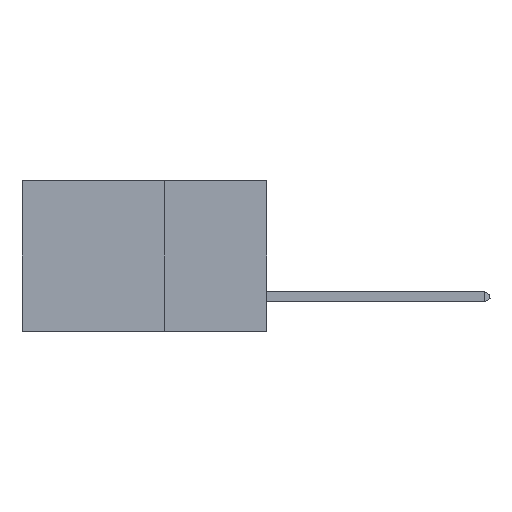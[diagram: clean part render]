
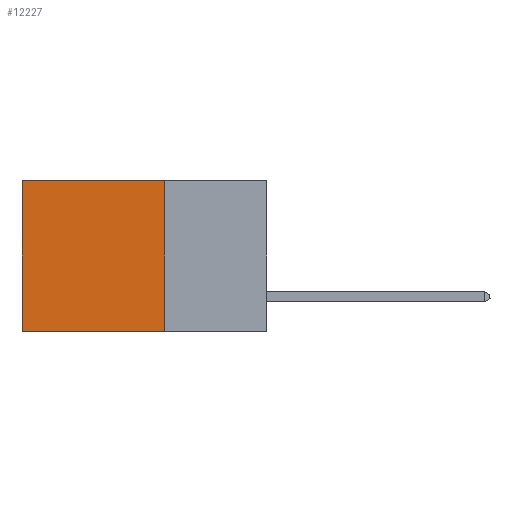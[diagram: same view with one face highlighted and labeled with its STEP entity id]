
A CAD part, left-side view. The second image highlights one B-rep face of the part: STEP entity #12227.
In plain terms, the highlighted planar face has unit normal (-1, 0, 0).
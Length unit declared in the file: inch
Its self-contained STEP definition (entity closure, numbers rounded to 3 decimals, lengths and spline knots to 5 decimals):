
#203 = ORIENTED_EDGE ( 'NONE', *, *, #2000, .F. ) ;
#1273 = ORIENTED_EDGE ( 'NONE', *, *, #4334, .T. ) ;
#1590 = VECTOR ( 'NONE', #4318, 39.37008 ) ;
#2000 = EDGE_CURVE ( 'NONE', #8468, #23145, #29877, .T. ) ;
#4318 = DIRECTION ( 'NONE',  ( 0., 1., 0. ) ) ;
#4334 = EDGE_CURVE ( 'NONE', #22499, #25801, #22245, .T. ) ;
#4381 = EDGE_LOOP ( 'NONE', ( #28928, #203, #22997, #1273 ) ) ;
#4832 = PLANE ( 'NONE',  #26429 ) ;
#5043 = VECTOR ( 'NONE', #27438, 39.37008 ) ;
#5474 = VECTOR ( 'NONE', #24535, 39.37008 ) ;
#6563 = CARTESIAN_POINT ( 'NONE',  ( 0.2875, 0.25, -0.37 ) ) ;
#7083 = DIRECTION ( 'NONE',  ( 0., 0., -1. ) ) ;
#8468 = VERTEX_POINT ( 'NONE', #30933 ) ;
#9014 = CARTESIAN_POINT ( 'NONE',  ( 0.2875, 0.6, -0.37 ) ) ;
#9348 = CARTESIAN_POINT ( 'NONE',  ( 0.2875, 0.25, 0. ) ) ;
#11976 = LINE ( 'NONE', #24220, #5474 ) ;
#12227 = ADVANCED_FACE ( 'NONE', ( #18623 ), #4832, .F. ) ;
#12377 = CARTESIAN_POINT ( 'NONE',  ( 0.2875, 0.25, 0. ) ) ;
#14038 = LINE ( 'NONE', #21580, #28235 ) ;
#14568 = EDGE_CURVE ( 'NONE', #22499, #8468, #11976, .T. ) ;
#15264 = CARTESIAN_POINT ( 'NONE',  ( 0.2875, 0.25, 0. ) ) ;
#16583 = EDGE_CURVE ( 'NONE', #25801, #23145, #14038, .T. ) ;
#18623 = FACE_OUTER_BOUND ( 'NONE', #4381, .T. ) ;
#21580 = CARTESIAN_POINT ( 'NONE',  ( 0.2875, 0.6, 0. ) ) ;
#22245 = LINE ( 'NONE', #12377, #5043 ) ;
#22499 = VERTEX_POINT ( 'NONE', #15264 ) ;
#22997 = ORIENTED_EDGE ( 'NONE', *, *, #14568, .F. ) ;
#23145 = VERTEX_POINT ( 'NONE', #9014 ) ;
#24220 = CARTESIAN_POINT ( 'NONE',  ( 0.2875, 0.25, 0. ) ) ;
#24535 = DIRECTION ( 'NONE',  ( 0., 0., -1. ) ) ;
#25192 = DIRECTION ( 'NONE',  ( 0., 0., -1. ) ) ;
#25801 = VERTEX_POINT ( 'NONE', #27856 ) ;
#26429 = AXIS2_PLACEMENT_3D ( 'NONE', #9348, #26432, #7083 ) ;
#26432 = DIRECTION ( 'NONE',  ( 1., 0., 0. ) ) ;
#27438 = DIRECTION ( 'NONE',  ( 0., 1., 0. ) ) ;
#27856 = CARTESIAN_POINT ( 'NONE',  ( 0.2875, 0.6, 0. ) ) ;
#28235 = VECTOR ( 'NONE', #25192, 39.37008 ) ;
#28928 = ORIENTED_EDGE ( 'NONE', *, *, #16583, .T. ) ;
#29877 = LINE ( 'NONE', #6563, #1590 ) ;
#30933 = CARTESIAN_POINT ( 'NONE',  ( 0.2875, 0.25, -0.37 ) ) ;
